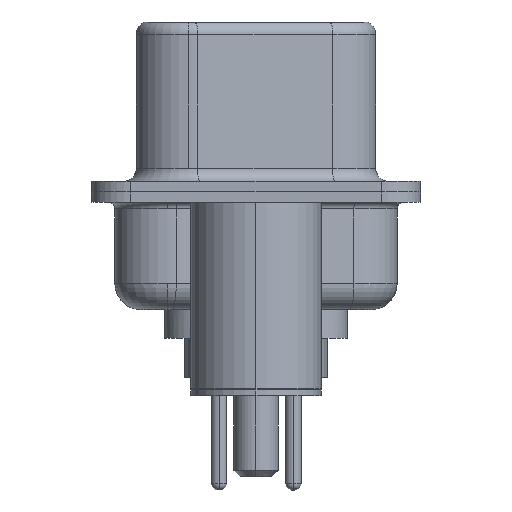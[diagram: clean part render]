
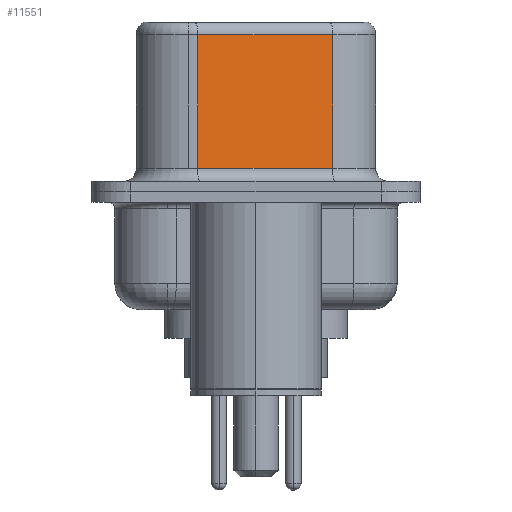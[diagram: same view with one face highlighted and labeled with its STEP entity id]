
A CAD part, left-side view. The second image highlights one B-rep face of the part: STEP entity #11551.
In plain terms, the highlighted planar face has unit normal (-0.985, -0.174, 0).
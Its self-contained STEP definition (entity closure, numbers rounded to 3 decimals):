
#556 = DIRECTION ( 'NONE',  ( 0.174, -0.985, 0. ) ) ;
#672 = EDGE_CURVE ( 'NONE', #15600, #7387, #19437, .T. ) ;
#1795 = CARTESIAN_POINT ( 'NONE',  ( 4.585, -2.927, 6.52 ) ) ;
#2369 = CARTESIAN_POINT ( 'NONE',  ( 4.585, -2.927, 0.9 ) ) ;
#3325 = EDGE_LOOP ( 'NONE', ( #11764, #13920, #7823, #7987 ) ) ;
#3633 = DIRECTION ( 'NONE',  ( 0., 0., -1. ) ) ;
#4189 = PLANE ( 'NONE',  #8570 ) ;
#4277 = LINE ( 'NONE', #14751, #18281 ) ;
#6385 = LINE ( 'NONE', #2369, #12383 ) ;
#7387 = VERTEX_POINT ( 'NONE', #23551 ) ;
#7585 = DIRECTION ( 'NONE',  ( -0.174, 0.985, 0. ) ) ;
#7823 = ORIENTED_EDGE ( 'NONE', *, *, #16046, .T. ) ;
#7987 = ORIENTED_EDGE ( 'NONE', *, *, #13411, .T. ) ;
#8570 = AXIS2_PLACEMENT_3D ( 'NONE', #11465, #16983, #18804 ) ;
#8835 = VERTEX_POINT ( 'NONE', #16002 ) ;
#9155 = CARTESIAN_POINT ( 'NONE',  ( 4.585, -2.927, 6.02 ) ) ;
#9968 = VECTOR ( 'NONE', #10963, 1000. ) ;
#10365 = EDGE_CURVE ( 'NONE', #15600, #8835, #15941, .T. ) ;
#10963 = DIRECTION ( 'NONE',  ( 0., 0., -1. ) ) ;
#11465 = CARTESIAN_POINT ( 'NONE',  ( 4.585, -2.927, 6.52 ) ) ;
#11551 = ADVANCED_FACE ( 'NONE', ( #22198 ), #4189, .F. ) ;
#11764 = ORIENTED_EDGE ( 'NONE', *, *, #672, .F. ) ;
#12383 = VECTOR ( 'NONE', #556, 1000. ) ;
#13411 = EDGE_CURVE ( 'NONE', #18506, #7387, #6385, .T. ) ;
#13920 = ORIENTED_EDGE ( 'NONE', *, *, #10365, .T. ) ;
#14751 = CARTESIAN_POINT ( 'NONE',  ( 3.675, 2.233, 6.52 ) ) ;
#15600 = VERTEX_POINT ( 'NONE', #23624 ) ;
#15941 = LINE ( 'NONE', #9155, #21091 ) ;
#16002 = CARTESIAN_POINT ( 'NONE',  ( 3.675, 2.233, 6.02 ) ) ;
#16046 = EDGE_CURVE ( 'NONE', #8835, #18506, #4277, .T. ) ;
#16983 = DIRECTION ( 'NONE',  ( 0.985, 0.174, 0. ) ) ;
#18281 = VECTOR ( 'NONE', #3633, 1000. ) ;
#18506 = VERTEX_POINT ( 'NONE', #23472 ) ;
#18804 = DIRECTION ( 'NONE',  ( -0.174, 0.985, 0. ) ) ;
#19437 = LINE ( 'NONE', #1795, #9968 ) ;
#21091 = VECTOR ( 'NONE', #7585, 1000. ) ;
#22198 = FACE_OUTER_BOUND ( 'NONE', #3325, .T. ) ;
#23472 = CARTESIAN_POINT ( 'NONE',  ( 3.675, 2.233, 0.9 ) ) ;
#23551 = CARTESIAN_POINT ( 'NONE',  ( 4.585, -2.927, 0.9 ) ) ;
#23624 = CARTESIAN_POINT ( 'NONE',  ( 4.585, -2.927, 6.02 ) ) ;
